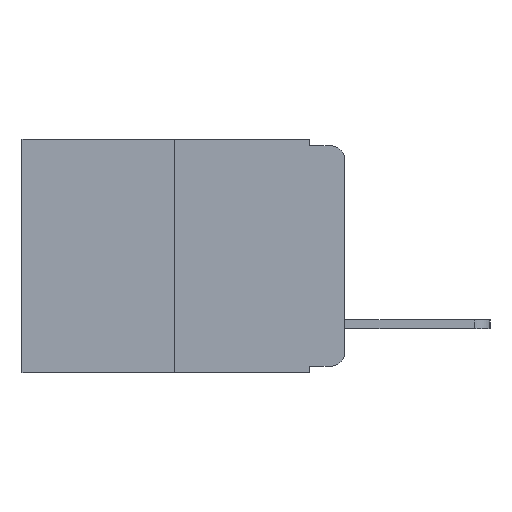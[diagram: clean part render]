
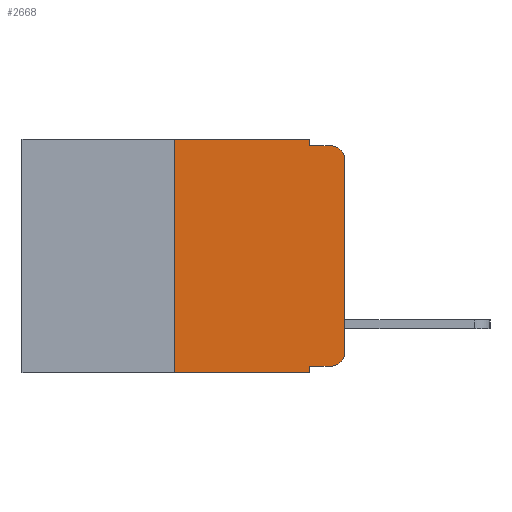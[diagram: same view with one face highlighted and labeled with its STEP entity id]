
A CAD part, left-side view. The second image highlights one B-rep face of the part: STEP entity #2668.
In plain terms, the highlighted planar face has unit normal (-1, 0, 0).
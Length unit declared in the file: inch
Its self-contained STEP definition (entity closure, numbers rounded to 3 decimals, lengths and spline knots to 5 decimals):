
#72 = ORIENTED_EDGE ( 'NONE', *, *, #9914, .T. ) ;
#181 = LINE ( 'NONE', #11177, #4412 ) ;
#238 = ORIENTED_EDGE ( 'NONE', *, *, #7844, .F. ) ;
#486 = CIRCLE ( 'NONE', #3613, 0.02 ) ;
#583 = ORIENTED_EDGE ( 'NONE', *, *, #10767, .F. ) ;
#731 = CARTESIAN_POINT ( 'NONE',  ( 0., 0.02, -0.313 ) ) ;
#754 = VERTEX_POINT ( 'NONE', #9672 ) ;
#758 = FACE_OUTER_BOUND ( 'NONE', #3222, .T. ) ;
#791 = EDGE_CURVE ( 'NONE', #6148, #2667, #8556, .T. ) ;
#930 = LINE ( 'NONE', #11185, #3430 ) ;
#1000 = ORIENTED_EDGE ( 'NONE', *, *, #3516, .F. ) ;
#1096 = DIRECTION ( 'NONE',  ( 0., 0., -1. ) ) ;
#1128 = VECTOR ( 'NONE', #1096, 39.37008 ) ;
#1229 = EDGE_CURVE ( 'NONE', #9990, #754, #11109, .T. ) ;
#1280 = CARTESIAN_POINT ( 'NONE',  ( 0., 0.051, -0.01 ) ) ;
#1469 = LINE ( 'NONE', #7765, #1128 ) ;
#1521 = PLANE ( 'NONE',  #5458 ) ;
#1619 = LINE ( 'NONE', #8115, #7967 ) ;
#1694 = CARTESIAN_POINT ( 'NONE',  ( 0., 0.051, -0.333 ) ) ;
#1786 = DIRECTION ( 'NONE',  ( 0., 0., -1. ) ) ;
#1876 = CARTESIAN_POINT ( 'NONE',  ( 0., 0.051, -0.343 ) ) ;
#2317 = ORIENTED_EDGE ( 'NONE', *, *, #5203, .F. ) ;
#2651 = ORIENTED_EDGE ( 'NONE', *, *, #1229, .T. ) ;
#2667 = VERTEX_POINT ( 'NONE', #4886 ) ;
#2668 = ADVANCED_FACE ( 'NONE', ( #758 ), #1521, .F. ) ;
#2870 = DIRECTION ( 'NONE',  ( 0., -1., 0. ) ) ;
#2938 = VECTOR ( 'NONE', #2870, 39.37008 ) ;
#3024 = DIRECTION ( 'NONE',  ( 0., -1., 0. ) ) ;
#3028 = CARTESIAN_POINT ( 'NONE',  ( 0., 0.051, -0.333 ) ) ;
#3222 = EDGE_LOOP ( 'NONE', ( #72, #4488, #1000, #238, #2317, #7308, #5970, #583, #2651, #7353 ) ) ;
#3270 = CIRCLE ( 'NONE', #3319, 0.02 ) ;
#3319 = AXIS2_PLACEMENT_3D ( 'NONE', #731, #7483, #1786 ) ;
#3332 = VERTEX_POINT ( 'NONE', #1876 ) ;
#3430 = VECTOR ( 'NONE', #6858, 39.37008 ) ;
#3516 = EDGE_CURVE ( 'NONE', #7929, #4873, #181, .T. ) ;
#3600 = DIRECTION ( 'NONE',  ( 1., 0., 0. ) ) ;
#3613 = AXIS2_PLACEMENT_3D ( 'NONE', #9544, #4274, #10424 ) ;
#3803 = VECTOR ( 'NONE', #12054, 39.37008 ) ;
#4173 = CARTESIAN_POINT ( 'NONE',  ( 0., 0., -0.313 ) ) ;
#4274 = DIRECTION ( 'NONE',  ( -1., 0., 0. ) ) ;
#4287 = DIRECTION ( 'NONE',  ( 0., 0., -1. ) ) ;
#4412 = VECTOR ( 'NONE', #11106, 39.37008 ) ;
#4488 = ORIENTED_EDGE ( 'NONE', *, *, #5577, .T. ) ;
#4543 = CARTESIAN_POINT ( 'NONE',  ( 0., 0.051, 0. ) ) ;
#4873 = VERTEX_POINT ( 'NONE', #7459 ) ;
#4886 = CARTESIAN_POINT ( 'NONE',  ( 0., 0.25, 0. ) ) ;
#5203 = EDGE_CURVE ( 'NONE', #2667, #7146, #6613, .T. ) ;
#5458 = AXIS2_PLACEMENT_3D ( 'NONE', #8462, #3600, #4287 ) ;
#5470 = DIRECTION ( 'NONE',  ( 0., 0., 1. ) ) ;
#5481 = LINE ( 'NONE', #5690, #2938 ) ;
#5575 = DIRECTION ( 'NONE',  ( 0., -1., 0. ) ) ;
#5577 = EDGE_CURVE ( 'NONE', #10897, #4873, #486, .T. ) ;
#5690 = CARTESIAN_POINT ( 'NONE',  ( 0., 0.473, -0.343 ) ) ;
#5970 = ORIENTED_EDGE ( 'NONE', *, *, #10556, .T. ) ;
#6148 = VERTEX_POINT ( 'NONE', #7889 ) ;
#6613 = LINE ( 'NONE', #12016, #8929 ) ;
#6858 = DIRECTION ( 'NONE',  ( 0., 0., -1. ) ) ;
#7146 = VERTEX_POINT ( 'NONE', #4543 ) ;
#7308 = ORIENTED_EDGE ( 'NONE', *, *, #791, .F. ) ;
#7353 = ORIENTED_EDGE ( 'NONE', *, *, #10548, .T. ) ;
#7459 = CARTESIAN_POINT ( 'NONE',  ( 0., 0.02, -0.01 ) ) ;
#7483 = DIRECTION ( 'NONE',  ( -1., 0., 0. ) ) ;
#7765 = CARTESIAN_POINT ( 'NONE',  ( 0., 0.051, 0. ) ) ;
#7837 = CARTESIAN_POINT ( 'NONE',  ( 0., 0., -0.03 ) ) ;
#7844 = EDGE_CURVE ( 'NONE', #7146, #7929, #1469, .T. ) ;
#7889 = CARTESIAN_POINT ( 'NONE',  ( 0., 0.25, -0.343 ) ) ;
#7929 = VERTEX_POINT ( 'NONE', #1280 ) ;
#7967 = VECTOR ( 'NONE', #5470, 39.37008 ) ;
#8115 = CARTESIAN_POINT ( 'NONE',  ( 0., 0., 0. ) ) ;
#8462 = CARTESIAN_POINT ( 'NONE',  ( 0., 0.473, 0. ) ) ;
#8543 = VECTOR ( 'NONE', #3024, 39.37008 ) ;
#8556 = LINE ( 'NONE', #10806, #3803 ) ;
#8929 = VECTOR ( 'NONE', #5575, 39.37008 ) ;
#9143 = VERTEX_POINT ( 'NONE', #4173 ) ;
#9544 = CARTESIAN_POINT ( 'NONE',  ( 0., 0.02, -0.03 ) ) ;
#9672 = CARTESIAN_POINT ( 'NONE',  ( 0., 0.02, -0.333 ) ) ;
#9914 = EDGE_CURVE ( 'NONE', #9143, #10897, #1619, .T. ) ;
#9990 = VERTEX_POINT ( 'NONE', #1694 ) ;
#10424 = DIRECTION ( 'NONE',  ( 0., 0., -1. ) ) ;
#10548 = EDGE_CURVE ( 'NONE', #754, #9143, #3270, .T. ) ;
#10556 = EDGE_CURVE ( 'NONE', #6148, #3332, #5481, .T. ) ;
#10767 = EDGE_CURVE ( 'NONE', #9990, #3332, #930, .T. ) ;
#10806 = CARTESIAN_POINT ( 'NONE',  ( 0., 0.25, 0. ) ) ;
#10897 = VERTEX_POINT ( 'NONE', #7837 ) ;
#11106 = DIRECTION ( 'NONE',  ( 0., -1., 0. ) ) ;
#11109 = LINE ( 'NONE', #3028, #8543 ) ;
#11177 = CARTESIAN_POINT ( 'NONE',  ( 0., 0.051, -0.01 ) ) ;
#11185 = CARTESIAN_POINT ( 'NONE',  ( 0., 0.051, 0. ) ) ;
#12016 = CARTESIAN_POINT ( 'NONE',  ( 0., 0.473, 0. ) ) ;
#12054 = DIRECTION ( 'NONE',  ( 0., 0., 1. ) ) ;
